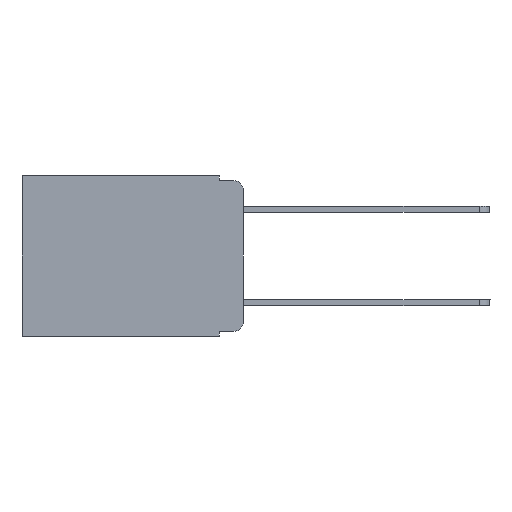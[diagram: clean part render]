
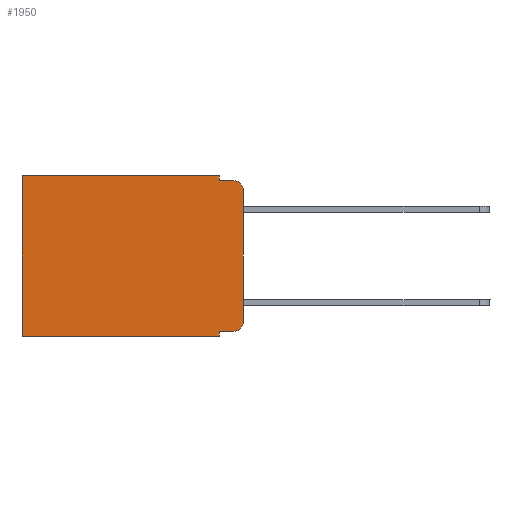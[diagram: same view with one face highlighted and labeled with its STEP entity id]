
A CAD part, left-side view. The second image highlights one B-rep face of the part: STEP entity #1950.
In plain terms, the highlighted planar face has unit normal (-1, 0, 0).
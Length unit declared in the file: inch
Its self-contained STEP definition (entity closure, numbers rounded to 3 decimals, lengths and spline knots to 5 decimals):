
#12 = EDGE_LOOP ( 'NONE', ( #9147, #11165, #8520, #8148, #10500, #5174, #2763, #9837, #5911, #1744 ) ) ;
#206 = CARTESIAN_POINT ( 'NONE',  ( 0.298, 0., -0.313 ) ) ;
#372 = VECTOR ( 'NONE', #6133, 39.37008 ) ;
#503 = EDGE_CURVE ( 'NONE', #3155, #7554, #8847, .T. ) ;
#615 = AXIS2_PLACEMENT_3D ( 'NONE', #3507, #11717, #5327 ) ;
#649 = LINE ( 'NONE', #6013, #7785 ) ;
#686 = DIRECTION ( 'NONE',  ( -1., 0., 0. ) ) ;
#908 = DIRECTION ( 'NONE',  ( 0., 0., -1. ) ) ;
#980 = FACE_OUTER_BOUND ( 'NONE', #12, .T. ) ;
#1050 = EDGE_CURVE ( 'NONE', #1438, #3136, #10829, .T. ) ;
#1438 = VERTEX_POINT ( 'NONE', #11681 ) ;
#1528 = VECTOR ( 'NONE', #5323, 39.37008 ) ;
#1744 = ORIENTED_EDGE ( 'NONE', *, *, #9064, .T. ) ;
#1950 = ADVANCED_FACE ( 'NONE', ( #980 ), #2648, .F. ) ;
#2108 = DIRECTION ( 'NONE',  ( 0., 1., 0. ) ) ;
#2356 = DIRECTION ( 'NONE',  ( 0., 0., -1. ) ) ;
#2467 = EDGE_CURVE ( 'NONE', #6154, #9016, #11215, .T. ) ;
#2648 = PLANE ( 'NONE',  #615 ) ;
#2763 = ORIENTED_EDGE ( 'NONE', *, *, #10183, .F. ) ;
#2945 = VERTEX_POINT ( 'NONE', #11744 ) ;
#3067 = LINE ( 'NONE', #4806, #6396 ) ;
#3136 = VERTEX_POINT ( 'NONE', #10308 ) ;
#3155 = VERTEX_POINT ( 'NONE', #7667 ) ;
#3507 = CARTESIAN_POINT ( 'NONE',  ( 0.298, 0., 0. ) ) ;
#3887 = CARTESIAN_POINT ( 'NONE',  ( 0.298, 0.02, -0.03 ) ) ;
#4173 = VERTEX_POINT ( 'NONE', #5795 ) ;
#4218 = VECTOR ( 'NONE', #11549, 39.37008 ) ;
#4523 = VECTOR ( 'NONE', #908, 39.37008 ) ;
#4806 = CARTESIAN_POINT ( 'NONE',  ( 0.298, 0., 0. ) ) ;
#5174 = ORIENTED_EDGE ( 'NONE', *, *, #5677, .T. ) ;
#5197 = EDGE_CURVE ( 'NONE', #6154, #4173, #10363, .T. ) ;
#5198 = CARTESIAN_POINT ( 'NONE',  ( 0.298, 0.051, -0.01 ) ) ;
#5323 = DIRECTION ( 'NONE',  ( 0., 0., -1. ) ) ;
#5327 = DIRECTION ( 'NONE',  ( 0., 0., -1. ) ) ;
#5602 = VECTOR ( 'NONE', #7346, 39.37008 ) ;
#5677 = EDGE_CURVE ( 'NONE', #4173, #6099, #7124, .T. ) ;
#5768 = AXIS2_PLACEMENT_3D ( 'NONE', #3887, #6700, #10445 ) ;
#5795 = CARTESIAN_POINT ( 'NONE',  ( 0.298, 0.473, 0. ) ) ;
#5911 = ORIENTED_EDGE ( 'NONE', *, *, #503, .T. ) ;
#6013 = CARTESIAN_POINT ( 'NONE',  ( 0.298, 0.051, 0. ) ) ;
#6058 = CARTESIAN_POINT ( 'NONE',  ( 0.298, 0.051, 0. ) ) ;
#6099 = VERTEX_POINT ( 'NONE', #9757 ) ;
#6133 = DIRECTION ( 'NONE',  ( 0., -1., 0. ) ) ;
#6154 = VERTEX_POINT ( 'NONE', #6058 ) ;
#6168 = CARTESIAN_POINT ( 'NONE',  ( 0.298, 0.02, -0.313 ) ) ;
#6396 = VECTOR ( 'NONE', #10257, 39.37008 ) ;
#6700 = DIRECTION ( 'NONE',  ( -1., 0., 0. ) ) ;
#7088 = EDGE_CURVE ( 'NONE', #3155, #2945, #649, .T. ) ;
#7124 = LINE ( 'NONE', #7268, #4523 ) ;
#7268 = CARTESIAN_POINT ( 'NONE',  ( 0.298, 0.473, 0. ) ) ;
#7346 = DIRECTION ( 'NONE',  ( 0., -1., 0. ) ) ;
#7378 = AXIS2_PLACEMENT_3D ( 'NONE', #6168, #686, #7987 ) ;
#7504 = LINE ( 'NONE', #7571, #9199 ) ;
#7554 = VERTEX_POINT ( 'NONE', #11093 ) ;
#7571 = CARTESIAN_POINT ( 'NONE',  ( 0.298, 0., -0.343 ) ) ;
#7649 = LINE ( 'NONE', #5198, #372 ) ;
#7667 = CARTESIAN_POINT ( 'NONE',  ( 0.298, 0.051, -0.333 ) ) ;
#7785 = VECTOR ( 'NONE', #2356, 39.37008 ) ;
#7789 = EDGE_CURVE ( 'NONE', #9016, #3136, #7649, .T. ) ;
#7820 = CIRCLE ( 'NONE', #7378, 0.02 ) ;
#7987 = DIRECTION ( 'NONE',  ( 0., 0., -1. ) ) ;
#8123 = CARTESIAN_POINT ( 'NONE',  ( 0.298, 0., 0. ) ) ;
#8148 = ORIENTED_EDGE ( 'NONE', *, *, #2467, .F. ) ;
#8179 = CARTESIAN_POINT ( 'NONE',  ( 0.298, 0.051, -0.333 ) ) ;
#8520 = ORIENTED_EDGE ( 'NONE', *, *, #7789, .F. ) ;
#8847 = LINE ( 'NONE', #8179, #5602 ) ;
#9016 = VERTEX_POINT ( 'NONE', #10624 ) ;
#9064 = EDGE_CURVE ( 'NONE', #7554, #9646, #7820, .T. ) ;
#9147 = ORIENTED_EDGE ( 'NONE', *, *, #9664, .F. ) ;
#9199 = VECTOR ( 'NONE', #2108, 39.37008 ) ;
#9646 = VERTEX_POINT ( 'NONE', #206 ) ;
#9664 = EDGE_CURVE ( 'NONE', #1438, #9646, #3067, .T. ) ;
#9757 = CARTESIAN_POINT ( 'NONE',  ( 0.298, 0.473, -0.343 ) ) ;
#9837 = ORIENTED_EDGE ( 'NONE', *, *, #7088, .F. ) ;
#10183 = EDGE_CURVE ( 'NONE', #2945, #6099, #7504, .T. ) ;
#10257 = DIRECTION ( 'NONE',  ( 0., 0., -1. ) ) ;
#10308 = CARTESIAN_POINT ( 'NONE',  ( 0.298, 0.02, -0.01 ) ) ;
#10363 = LINE ( 'NONE', #8123, #4218 ) ;
#10445 = DIRECTION ( 'NONE',  ( 0., 0., -1. ) ) ;
#10500 = ORIENTED_EDGE ( 'NONE', *, *, #5197, .T. ) ;
#10624 = CARTESIAN_POINT ( 'NONE',  ( 0.298, 0.051, -0.01 ) ) ;
#10718 = CARTESIAN_POINT ( 'NONE',  ( 0.298, 0.051, 0. ) ) ;
#10829 = CIRCLE ( 'NONE', #5768, 0.02 ) ;
#11093 = CARTESIAN_POINT ( 'NONE',  ( 0.298, 0.02, -0.333 ) ) ;
#11165 = ORIENTED_EDGE ( 'NONE', *, *, #1050, .T. ) ;
#11215 = LINE ( 'NONE', #10718, #1528 ) ;
#11549 = DIRECTION ( 'NONE',  ( 0., 1., 0. ) ) ;
#11681 = CARTESIAN_POINT ( 'NONE',  ( 0.298, 0., -0.03 ) ) ;
#11717 = DIRECTION ( 'NONE',  ( 1., 0., 0. ) ) ;
#11744 = CARTESIAN_POINT ( 'NONE',  ( 0.298, 0.051, -0.343 ) ) ;
